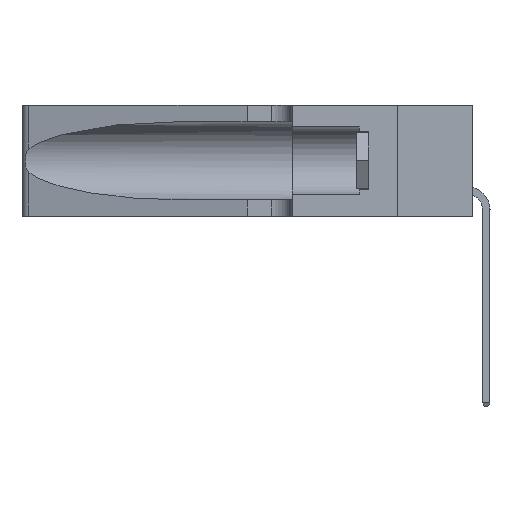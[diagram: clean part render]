
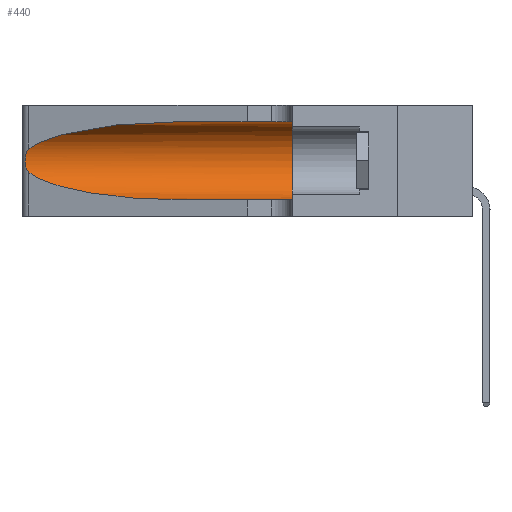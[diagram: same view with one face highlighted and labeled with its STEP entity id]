
A CAD part, left-side view. The second image highlights one B-rep face of the part: STEP entity #440.
In plain terms, the highlighted cylindrical face has radius 3.308 mm (diameter 6.617 mm), a partial arc.
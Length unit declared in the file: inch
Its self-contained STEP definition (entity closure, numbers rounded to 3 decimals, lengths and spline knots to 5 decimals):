
#440 = ADVANCED_FACE ( 'NONE', ( #10674 ), #16105, .F. ) ;
#883 = CARTESIAN_POINT ( 'NONE',  ( 0.1305, 1.61858, 0.05475 ) ) ;
#1225 = CARTESIAN_POINT ( 'NONE',  ( 0.1305, 1.61858, 0.185 ) ) ;
#2753 = CARTESIAN_POINT ( 'NONE',  ( 0.25639, 1.23186, 0.15144 ) ) ;
#2803 = DIRECTION ( 'NONE',  ( 0., -1., 0. ) ) ;
#3869 = VERTEX_POINT ( 'NONE', #10436 ) ;
#4169 = CARTESIAN_POINT ( 'NONE',  ( 0.25487, 1.22718, 0.14631 ) ) ;
#6474 = EDGE_CURVE ( 'NONE', #50465, #15507, #35625, .T. ) ;
#6692 = CARTESIAN_POINT ( 'NONE',  ( 0.25555, 1.22993, 0.14849 ) ) ;
#6696 = LINE ( 'NONE', #15405, #15279 ) ;
#6827 = EDGE_CURVE ( 'NONE', #11683, #15507, #50263, .T. ) ;
#7092 = CARTESIAN_POINT ( 'NONE',  ( 0.1305, 0.35, 0.185 ) ) ;
#8259 = VERTEX_POINT ( 'NONE', #22313 ) ;
#8559 = ORIENTED_EDGE ( 'NONE', *, *, #25134, .T. ) ;
#10436 = CARTESIAN_POINT ( 'NONE',  ( 0.25487, 1.22718, 0.14631 ) ) ;
#10674 = FACE_OUTER_BOUND ( 'NONE', #40368, .T. ) ;
#11683 = VERTEX_POINT ( 'NONE', #30128 ) ;
#12169 = VERTEX_POINT ( 'NONE', #25640 ) ;
#12390 = VECTOR ( 'NONE', #2803, 39.37008 ) ;
#12764 = DIRECTION ( 'NONE',  ( 0., -1., 0. ) ) ;
#14703 = CARTESIAN_POINT ( 'NONE',  ( 0.2373, 1.15595, 0.28018 ) ) ;
#15279 = VECTOR ( 'NONE', #47197, 39.37008 ) ;
#15405 = CARTESIAN_POINT ( 'NONE',  ( 0.1305, 1.61858, 0.31525 ) ) ;
#15507 = VERTEX_POINT ( 'NONE', #48249 ) ;
#16105 = CYLINDRICAL_SURFACE ( 'NONE', #19765, 0.13025 ) ;
#16543 = CARTESIAN_POINT ( 'NONE',  ( 0.25487, 1.22718, 0.22369 ) ) ;
#17582 = CARTESIAN_POINT ( 'NONE',  ( 0.25639, 1.23184, 0.21858 ) ) ;
#18150 = CARTESIAN_POINT ( 'NONE',  ( 0.26017, 1.23833, 0.17102 ) ) ;
#18397 = CARTESIAN_POINT ( 'NONE',  ( 0.2373, 1.15595, 0.08982 ) ) ;
#18625 = ORIENTED_EDGE ( 'NONE', *, *, #46751, .T. ) ;
#19017 = AXIS2_PLACEMENT_3D ( 'NONE', #7092, #42233, #34779 ) ;
#19723 =( BOUNDED_CURVE ( )  B_SPLINE_CURVE ( 3, ( #38430, #34862, #14703, #22618 ),
 .UNSPECIFIED., .F., .T. ) 
 B_SPLINE_CURVE_WITH_KNOTS ( ( 4, 4 ),
 ( 1.5708, 2.84003 ),
 .UNSPECIFIED. ) 
 CURVE ( )  GEOMETRIC_REPRESENTATION_ITEM ( )  RATIONAL_B_SPLINE_CURVE ( ( 1., 0.87, 0.87, 1. ) ) 
 REPRESENTATION_ITEM ( '' )  );
#19765 = AXIS2_PLACEMENT_3D ( 'NONE', #1225, #12764, #36658 ) ;
#21685 = EDGE_CURVE ( 'NONE', #8259, #50465, #6696, .T. ) ;
#21912 = CARTESIAN_POINT ( 'NONE',  ( 0.25787, 1.23484, 0.2124 ) ) ;
#22313 = CARTESIAN_POINT ( 'NONE',  ( 0.1305, 0.72297, 0.31525 ) ) ;
#22362 = CARTESIAN_POINT ( 'NONE',  ( 0.18966, 0.96281, 0.05475 ) ) ;
#22618 = CARTESIAN_POINT ( 'NONE',  ( 0.25487, 1.22718, 0.22369 ) ) ;
#22640 = CARTESIAN_POINT ( 'NONE',  ( 0.26075, 1.23896, 0.19203 ) ) ;
#25134 = EDGE_CURVE ( 'NONE', #12169, #3869, #27555, .T. ) ;
#25640 = CARTESIAN_POINT ( 'NONE',  ( 0.25487, 1.22718, 0.22369 ) ) ;
#26041 = CARTESIAN_POINT ( 'NONE',  ( 0.25856, 1.23593, 0.16098 ) ) ;
#27555 = B_SPLINE_CURVE_WITH_KNOTS ( 'NONE', 3,
 ( #16543, #28348, #17582, #21912, #29392, #44834, #22640, #30152, #18150, #26041, #34389, #2753, #6692, #4169 ),
 .UNSPECIFIED., .F., .F.,
 ( 4, 2, 2, 2, 2, 2, 4 ),
 ( 0., 0.00027, 0.00053, 0.00107, 0.0016, 0.00187, 0.00214 ),
 .UNSPECIFIED. ) ;
#28348 = CARTESIAN_POINT ( 'NONE',  ( 0.25555, 1.22994, 0.2215 ) ) ;
#29392 = CARTESIAN_POINT ( 'NONE',  ( 0.25854, 1.2359, 0.20912 ) ) ;
#29759 =( BOUNDED_CURVE ( )  B_SPLINE_CURVE ( 3, ( #41366, #18397, #22362, #33403 ),
 .UNSPECIFIED., .F., .T. ) 
 B_SPLINE_CURVE_WITH_KNOTS ( ( 4, 4 ),
 ( 3.44316, 4.71239 ),
 .UNSPECIFIED. ) 
 CURVE ( )  GEOMETRIC_REPRESENTATION_ITEM ( )  RATIONAL_B_SPLINE_CURVE ( ( 1., 0.87, 0.87, 1. ) ) 
 REPRESENTATION_ITEM ( '' )  );
#30128 = CARTESIAN_POINT ( 'NONE',  ( 0.1305, 0.72297, 0.05475 ) ) ;
#30152 = CARTESIAN_POINT ( 'NONE',  ( 0.26075, 1.23896, 0.178 ) ) ;
#33403 = CARTESIAN_POINT ( 'NONE',  ( 0.1305, 0.72297, 0.05475 ) ) ;
#33494 = ORIENTED_EDGE ( 'NONE', *, *, #21685, .F. ) ;
#34389 = CARTESIAN_POINT ( 'NONE',  ( 0.25789, 1.23486, 0.15765 ) ) ;
#34508 = ORIENTED_EDGE ( 'NONE', *, *, #49827, .T. ) ;
#34779 = DIRECTION ( 'NONE',  ( 0., 0., 1. ) ) ;
#34862 = CARTESIAN_POINT ( 'NONE',  ( 0.18966, 0.96281, 0.31525 ) ) ;
#35625 = CIRCLE ( 'NONE', #19017, 0.13025 ) ;
#36658 = DIRECTION ( 'NONE',  ( 0., 0., -1. ) ) ;
#38430 = CARTESIAN_POINT ( 'NONE',  ( 0.1305, 0.72297, 0.31525 ) ) ;
#39957 = ORIENTED_EDGE ( 'NONE', *, *, #6827, .T. ) ;
#40368 = EDGE_LOOP ( 'NONE', ( #18625, #8559, #34508, #39957, #47193, #33494 ) ) ;
#41366 = CARTESIAN_POINT ( 'NONE',  ( 0.25487, 1.22718, 0.14631 ) ) ;
#42233 = DIRECTION ( 'NONE',  ( 0., 1., 0. ) ) ;
#42698 = CARTESIAN_POINT ( 'NONE',  ( 0.1305, 0.35, 0.31525 ) ) ;
#44834 = CARTESIAN_POINT ( 'NONE',  ( 0.26018, 1.23835, 0.19895 ) ) ;
#46751 = EDGE_CURVE ( 'NONE', #8259, #12169, #19723, .T. ) ;
#47193 = ORIENTED_EDGE ( 'NONE', *, *, #6474, .F. ) ;
#47197 = DIRECTION ( 'NONE',  ( 0., -1., 0. ) ) ;
#48249 = CARTESIAN_POINT ( 'NONE',  ( 0.1305, 0.35, 0.05475 ) ) ;
#49827 = EDGE_CURVE ( 'NONE', #3869, #11683, #29759, .T. ) ;
#50263 = LINE ( 'NONE', #883, #12390 ) ;
#50465 = VERTEX_POINT ( 'NONE', #42698 ) ;
